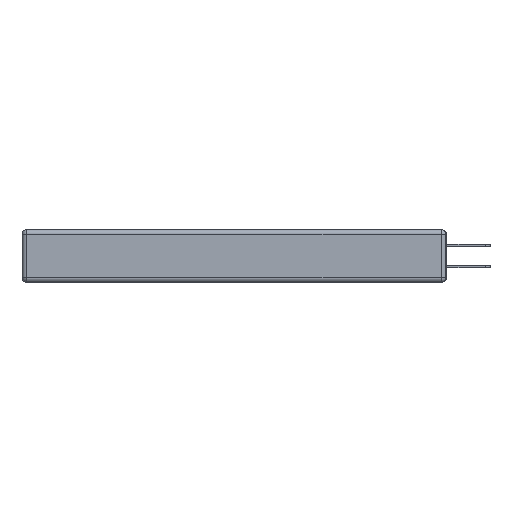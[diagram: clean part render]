
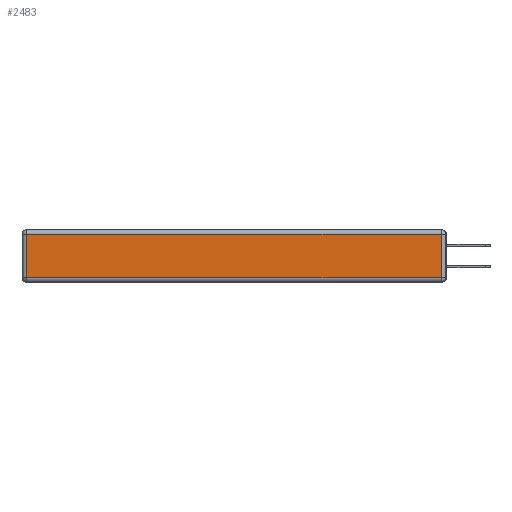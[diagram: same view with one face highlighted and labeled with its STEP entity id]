
A CAD part, left-side view. The second image highlights one B-rep face of the part: STEP entity #2483.
In plain terms, the highlighted planar face has unit normal (-1, 0, 0).
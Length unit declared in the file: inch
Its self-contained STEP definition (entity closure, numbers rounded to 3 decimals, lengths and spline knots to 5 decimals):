
#502 = VECTOR ( 'NONE', #18425, 39.37008 ) ;
#1002 = DIRECTION ( 'NONE',  ( 0., 1., 0. ) ) ;
#1086 = DIRECTION ( 'NONE',  ( -1., 0., 0. ) ) ;
#1492 = LINE ( 'NONE', #11965, #19378 ) ;
#1609 = DIRECTION ( 'NONE',  ( 0., 0., -1. ) ) ;
#1988 = CARTESIAN_POINT ( 'NONE',  ( 0., 2.72, -0.313 ) ) ;
#2332 = ORIENTED_EDGE ( 'NONE', *, *, #9403, .T. ) ;
#2396 = CARTESIAN_POINT ( 'NONE',  ( 0., 0.03, -0.313 ) ) ;
#2432 = EDGE_LOOP ( 'NONE', ( #2332, #5857, #3727, #14127 ) ) ;
#2483 = ADVANCED_FACE ( 'NONE', ( #15444 ), #10080, .T. ) ;
#2927 = VERTEX_POINT ( 'NONE', #1988 ) ;
#3101 = VECTOR ( 'NONE', #1002, 39.37008 ) ;
#3727 = ORIENTED_EDGE ( 'NONE', *, *, #10368, .T. ) ;
#4478 = DIRECTION ( 'NONE',  ( 0., -1., 0. ) ) ;
#4485 = LINE ( 'NONE', #7908, #502 ) ;
#4963 = LINE ( 'NONE', #10542, #11768 ) ;
#5384 = CARTESIAN_POINT ( 'NONE',  ( 0., 2.75, -0.03 ) ) ;
#5769 = EDGE_CURVE ( 'NONE', #18335, #7726, #4485, .T. ) ;
#5857 = ORIENTED_EDGE ( 'NONE', *, *, #5769, .T. ) ;
#7491 = CARTESIAN_POINT ( 'NONE',  ( 0., 2.72, -0.03 ) ) ;
#7726 = VERTEX_POINT ( 'NONE', #10379 ) ;
#7908 = CARTESIAN_POINT ( 'NONE',  ( 0., 0.03, -0.343 ) ) ;
#9403 = EDGE_CURVE ( 'NONE', #2927, #18335, #1492, .T. ) ;
#10080 = PLANE ( 'NONE',  #17731 ) ;
#10368 = EDGE_CURVE ( 'NONE', #7726, #18461, #12743, .T. ) ;
#10379 = CARTESIAN_POINT ( 'NONE',  ( 0., 0.03, -0.03 ) ) ;
#10542 = CARTESIAN_POINT ( 'NONE',  ( 0., 2.72, -0.343 ) ) ;
#11655 = DIRECTION ( 'NONE',  ( 0., 0., 1. ) ) ;
#11768 = VECTOR ( 'NONE', #1609, 39.37008 ) ;
#11890 = EDGE_CURVE ( 'NONE', #18461, #2927, #4963, .T. ) ;
#11965 = CARTESIAN_POINT ( 'NONE',  ( 0., 0., -0.313 ) ) ;
#12743 = LINE ( 'NONE', #5384, #3101 ) ;
#13205 = CARTESIAN_POINT ( 'NONE',  ( 0., 0., -0.343 ) ) ;
#14127 = ORIENTED_EDGE ( 'NONE', *, *, #11890, .T. ) ;
#15444 = FACE_OUTER_BOUND ( 'NONE', #2432, .T. ) ;
#17731 = AXIS2_PLACEMENT_3D ( 'NONE', #13205, #1086, #11655 ) ;
#18335 = VERTEX_POINT ( 'NONE', #2396 ) ;
#18425 = DIRECTION ( 'NONE',  ( 0., 0., 1. ) ) ;
#18461 = VERTEX_POINT ( 'NONE', #7491 ) ;
#19378 = VECTOR ( 'NONE', #4478, 39.37008 ) ;
